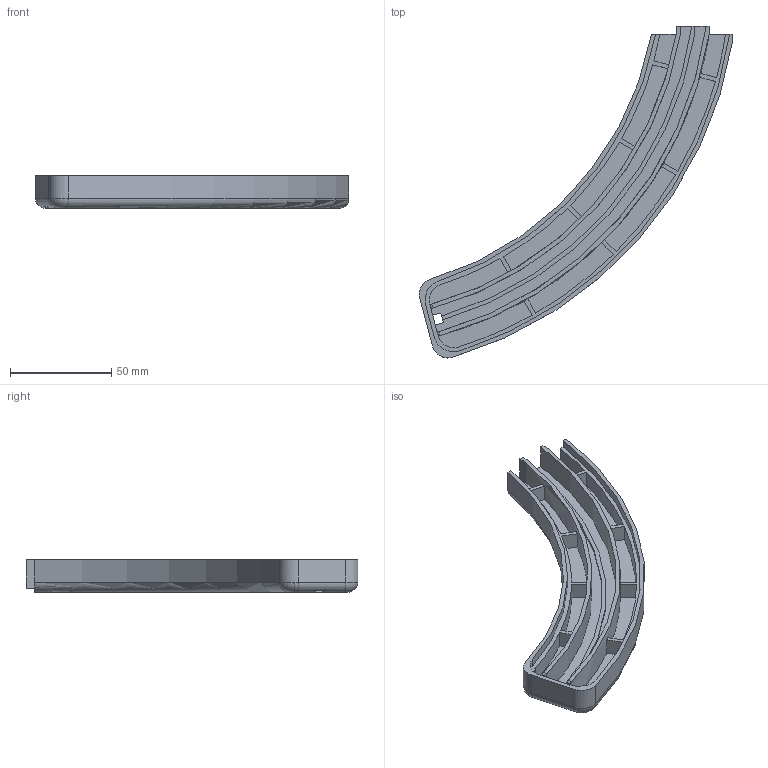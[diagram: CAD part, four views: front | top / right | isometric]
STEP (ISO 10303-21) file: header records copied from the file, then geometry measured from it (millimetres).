
FILE_DESCRIPTION (( 'STEP AP214' ), '1' );
FILE_NAME ('left_large.STEP', '2013-07-01T00:23:58', ( '' ), ( '' ), 'SwSTEP 2.0', 'SolidWorks 2013', '' );
FILE_SCHEMA (( 'AUTOMOTIVE_DESIGN' ));
Length unit declared in the file: millimetre
Products named in the file (1): left_large
Bounding box: 154.47 x 163.55 x 16 mm (x, y, z)
Volume: 59340.7 mm3; surface area: 39065.8 mm2
Topology: 1 solids, 1 shells, 87 faces, 252 edges, 165 vertices
Faces by surface type: plane 53, cylinder 29, torus 5
Entity records: 2973 total; most frequent: CARTESIAN_POINT 578, ORIENTED_EDGE 504, DIRECTION 503, EDGE_CURVE 252, AXIS2_PLACEMENT_3D 170, VERTEX_POINT 165, LINE 163, VECTOR 163
